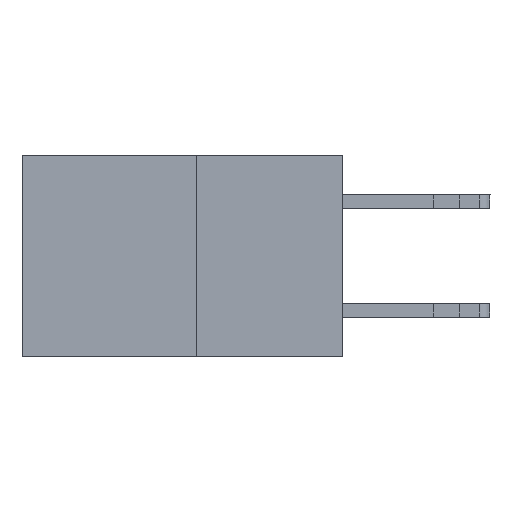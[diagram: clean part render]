
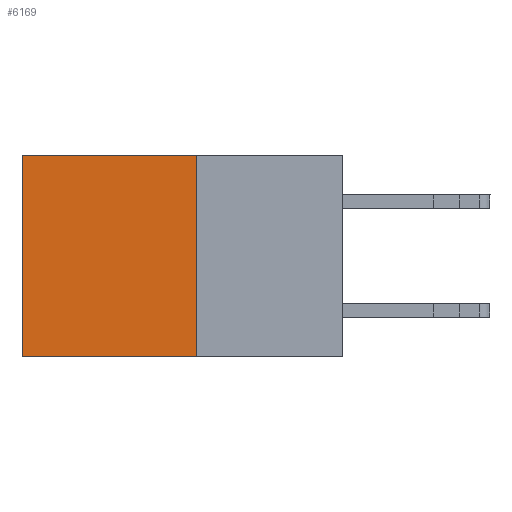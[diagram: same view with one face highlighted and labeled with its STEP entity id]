
A CAD part, left-side view. The second image highlights one B-rep face of the part: STEP entity #6169.
In plain terms, the highlighted planar face has unit normal (-1, 0, 0).
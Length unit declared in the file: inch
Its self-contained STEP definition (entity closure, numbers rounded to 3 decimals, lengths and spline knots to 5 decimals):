
#929 = CARTESIAN_POINT ( 'NONE',  ( 0.277, 0.27, 0. ) ) ;
#930 = CARTESIAN_POINT ( 'NONE',  ( 0.277, 0.59, 0. ) ) ;
#1832 = VERTEX_POINT ( 'NONE', #18697 ) ;
#1872 = LINE ( 'NONE', #6482, #7904 ) ;
#2317 = ORIENTED_EDGE ( 'NONE', *, *, #20134, .F. ) ;
#2883 = EDGE_CURVE ( 'NONE', #5249, #14662, #1872, .T. ) ;
#3476 = CARTESIAN_POINT ( 'NONE',  ( 0.277, 0.27, -0.37 ) ) ;
#3540 = VECTOR ( 'NONE', #11383, 39.37008 ) ;
#4093 = AXIS2_PLACEMENT_3D ( 'NONE', #13222, #13121, #15996 ) ;
#5226 = VECTOR ( 'NONE', #16031, 39.37008 ) ;
#5249 = VERTEX_POINT ( 'NONE', #929 ) ;
#5379 = ORIENTED_EDGE ( 'NONE', *, *, #17593, .T. ) ;
#6169 = ADVANCED_FACE ( 'NONE', ( #9769 ), #16302, .F. ) ;
#6482 = CARTESIAN_POINT ( 'NONE',  ( 0.277, 0.27, -0.37 ) ) ;
#7769 = VECTOR ( 'NONE', #12324, 39.37008 ) ;
#7851 = LINE ( 'NONE', #9067, #7769 ) ;
#7904 = VECTOR ( 'NONE', #18930, 39.37008 ) ;
#8041 = CARTESIAN_POINT ( 'NONE',  ( 0.277, 0.59, -0.37 ) ) ;
#8308 = LINE ( 'NONE', #11356, #5226 ) ;
#9067 = CARTESIAN_POINT ( 'NONE',  ( 0.277, 0.27, 0. ) ) ;
#9769 = FACE_OUTER_BOUND ( 'NONE', #19933, .T. ) ;
#10096 = ORIENTED_EDGE ( 'NONE', *, *, #2883, .F. ) ;
#11356 = CARTESIAN_POINT ( 'NONE',  ( 0.277, 0.27, -0.37 ) ) ;
#11383 = DIRECTION ( 'NONE',  ( 0., 0., -1. ) ) ;
#12324 = DIRECTION ( 'NONE',  ( 0., 1., 0. ) ) ;
#13121 = DIRECTION ( 'NONE',  ( 1., 0., 0. ) ) ;
#13222 = CARTESIAN_POINT ( 'NONE',  ( 0.277, 0.27, -0.37 ) ) ;
#14662 = VERTEX_POINT ( 'NONE', #3476 ) ;
#15996 = DIRECTION ( 'NONE',  ( 0., 0., -1. ) ) ;
#16031 = DIRECTION ( 'NONE',  ( 0., 1., 0. ) ) ;
#16302 = PLANE ( 'NONE',  #4093 ) ;
#17593 = EDGE_CURVE ( 'NONE', #18080, #1832, #19061, .T. ) ;
#17794 = EDGE_CURVE ( 'NONE', #5249, #18080, #7851, .T. ) ;
#18080 = VERTEX_POINT ( 'NONE', #930 ) ;
#18697 = CARTESIAN_POINT ( 'NONE',  ( 0.277, 0.59, -0.37 ) ) ;
#18849 = ORIENTED_EDGE ( 'NONE', *, *, #17794, .T. ) ;
#18930 = DIRECTION ( 'NONE',  ( 0., 0., -1. ) ) ;
#19061 = LINE ( 'NONE', #8041, #3540 ) ;
#19933 = EDGE_LOOP ( 'NONE', ( #5379, #2317, #10096, #18849 ) ) ;
#20134 = EDGE_CURVE ( 'NONE', #14662, #1832, #8308, .T. ) ;
